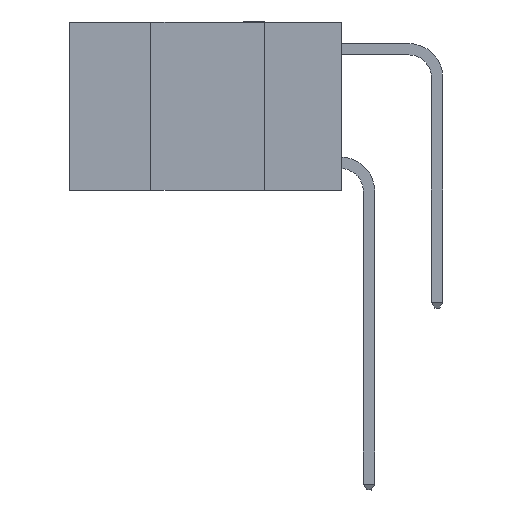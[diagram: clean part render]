
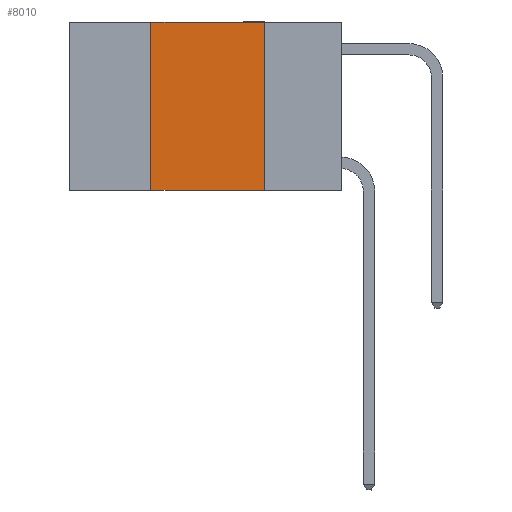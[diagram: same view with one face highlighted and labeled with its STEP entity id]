
A CAD part, left-side view. The second image highlights one B-rep face of the part: STEP entity #8010.
In plain terms, the highlighted planar face has unit normal (-1, 0, 0).
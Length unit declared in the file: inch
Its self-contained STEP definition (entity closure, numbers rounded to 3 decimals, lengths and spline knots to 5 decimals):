
#221 = VERTEX_POINT ( 'NONE', #13890 ) ;
#484 = VERTEX_POINT ( 'NONE', #9757 ) ;
#537 = PLANE ( 'NONE',  #10479 ) ;
#612 = VECTOR ( 'NONE', #10004, 39.37008 ) ;
#1844 = LINE ( 'NONE', #7539, #9147 ) ;
#2579 = VECTOR ( 'NONE', #6912, 39.37008 ) ;
#4133 = ORIENTED_EDGE ( 'NONE', *, *, #4902, .F. ) ;
#4165 = EDGE_CURVE ( 'NONE', #484, #221, #13624, .T. ) ;
#4902 = EDGE_CURVE ( 'NONE', #7792, #5893, #1844, .T. ) ;
#5055 = VECTOR ( 'NONE', #10457, 39.37008 ) ;
#5106 = EDGE_CURVE ( 'NONE', #484, #5893, #13110, .T. ) ;
#5231 = DIRECTION ( 'NONE',  ( 0., 0., -1. ) ) ;
#5269 = FACE_OUTER_BOUND ( 'NONE', #8108, .T. ) ;
#5529 = ORIENTED_EDGE ( 'NONE', *, *, #5106, .T. ) ;
#5893 = VERTEX_POINT ( 'NONE', #9047 ) ;
#6180 = ORIENTED_EDGE ( 'NONE', *, *, #9159, .F. ) ;
#6224 = DIRECTION ( 'NONE',  ( 1., 0., 0. ) ) ;
#6241 = CARTESIAN_POINT ( 'NONE',  ( 0., 0.6, 0. ) ) ;
#6639 = LINE ( 'NONE', #6241, #5055 ) ;
#6912 = DIRECTION ( 'NONE',  ( 0., 0., 1. ) ) ;
#7191 = CARTESIAN_POINT ( 'NONE',  ( 0., 0.17, 0. ) ) ;
#7539 = CARTESIAN_POINT ( 'NONE',  ( 0., 0.17, 0. ) ) ;
#7792 = VERTEX_POINT ( 'NONE', #7191 ) ;
#8010 = ADVANCED_FACE ( 'NONE', ( #5269 ), #537, .F. ) ;
#8108 = EDGE_LOOP ( 'NONE', ( #4133, #6180, #9717, #5529 ) ) ;
#8333 = CARTESIAN_POINT ( 'NONE',  ( 0., 0.6, 0. ) ) ;
#9047 = CARTESIAN_POINT ( 'NONE',  ( 0., 0.17, -0.37 ) ) ;
#9147 = VECTOR ( 'NONE', #13060, 39.37008 ) ;
#9159 = EDGE_CURVE ( 'NONE', #221, #7792, #6639, .T. ) ;
#9717 = ORIENTED_EDGE ( 'NONE', *, *, #4165, .F. ) ;
#9757 = CARTESIAN_POINT ( 'NONE',  ( 0., 0.42, -0.37 ) ) ;
#10004 = DIRECTION ( 'NONE',  ( 0., -1., 0. ) ) ;
#10053 = CARTESIAN_POINT ( 'NONE',  ( 0., 0.6, -0.37 ) ) ;
#10173 = CARTESIAN_POINT ( 'NONE',  ( 0., 0.42, 0. ) ) ;
#10457 = DIRECTION ( 'NONE',  ( 0., -1., 0. ) ) ;
#10479 = AXIS2_PLACEMENT_3D ( 'NONE', #8333, #6224, #5231 ) ;
#13060 = DIRECTION ( 'NONE',  ( 0., 0., -1. ) ) ;
#13110 = LINE ( 'NONE', #10053, #612 ) ;
#13624 = LINE ( 'NONE', #10173, #2579 ) ;
#13890 = CARTESIAN_POINT ( 'NONE',  ( 0., 0.42, 0. ) ) ;
